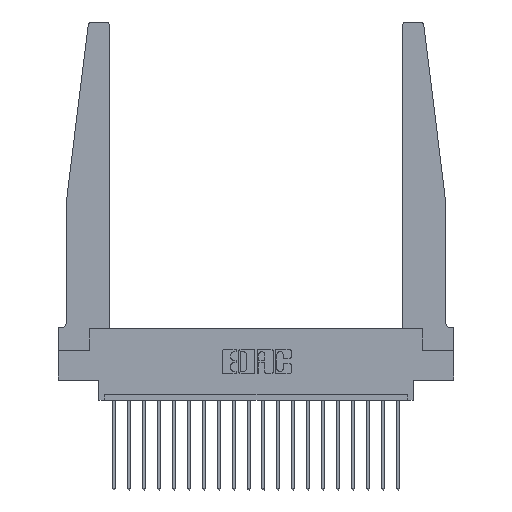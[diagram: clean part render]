
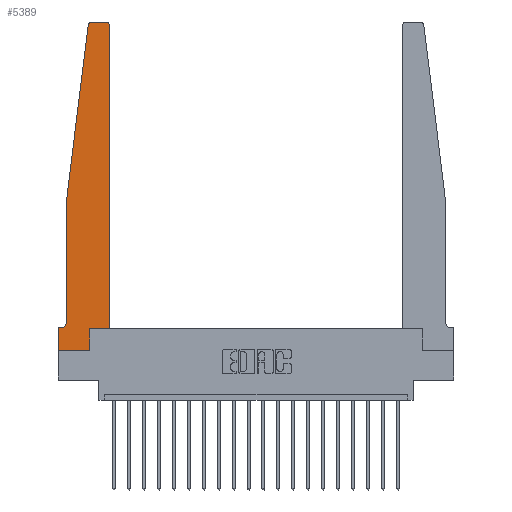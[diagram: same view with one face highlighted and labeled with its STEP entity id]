
A CAD part, top view. The second image highlights one B-rep face of the part: STEP entity #5389.
In plain terms, the highlighted planar face has unit normal (0, 0, 1).
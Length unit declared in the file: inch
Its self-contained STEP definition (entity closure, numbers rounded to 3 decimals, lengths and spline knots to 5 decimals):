
#49 = VERTEX_POINT ( 'NONE', #6301 ) ;
#795 = CARTESIAN_POINT ( 'NONE',  ( 0.425, 0.18, 0.37 ) ) ;
#1179 = CARTESIAN_POINT ( 'NONE',  ( 0.27653, 2.72, 0.37 ) ) ;
#1260 = EDGE_CURVE ( 'NONE', #10185, #16348, #17392, .T. ) ;
#1673 = ORIENTED_EDGE ( 'NONE', *, *, #4589, .T. ) ;
#1881 = CARTESIAN_POINT ( 'NONE',  ( 0., 0.1875, 0.37 ) ) ;
#1901 = DIRECTION ( 'NONE',  ( 1., 0., 0. ) ) ;
#2893 = ORIENTED_EDGE ( 'NONE', *, *, #15135, .T. ) ;
#2908 = ORIENTED_EDGE ( 'NONE', *, *, #1260, .T. ) ;
#3196 = CARTESIAN_POINT ( 'NONE',  ( 0.065, 0.1875, 0.37 ) ) ;
#3434 = DIRECTION ( 'NONE',  ( 1., 0., 0. ) ) ;
#3509 = EDGE_CURVE ( 'NONE', #18411, #6679, #15982, .T. ) ;
#3593 = CARTESIAN_POINT ( 'NONE',  ( 0.395, 2.72, 0.37 ) ) ;
#3826 = AXIS2_PLACEMENT_3D ( 'NONE', #6057, #15390, #5796 ) ;
#3918 = CARTESIAN_POINT ( 'NONE',  ( 0.2605, 0.18, 0.37 ) ) ;
#3995 = ORIENTED_EDGE ( 'NONE', *, *, #15138, .T. ) ;
#4188 = VECTOR ( 'NONE', #19390, 39.37008 ) ;
#4202 = ORIENTED_EDGE ( 'NONE', *, *, #13444, .T. ) ;
#4589 = EDGE_CURVE ( 'NONE', #14810, #14630, #9837, .T. ) ;
#4624 = EDGE_CURVE ( 'NONE', #17003, #15320, #13993, .T. ) ;
#4866 = CARTESIAN_POINT ( 'NONE',  ( 0.065, 1.25, 0.37 ) ) ;
#5377 = FACE_OUTER_BOUND ( 'NONE', #11152, .T. ) ;
#5389 = ADVANCED_FACE ( 'NONE', ( #5377 ), #9678, .T. ) ;
#5394 = DIRECTION ( 'NONE',  ( 0., 1., 0. ) ) ;
#5549 = ORIENTED_EDGE ( 'NONE', *, *, #12049, .T. ) ;
#5648 = CARTESIAN_POINT ( 'NONE',  ( 0.25, 2.75, 0.37 ) ) ;
#5796 = DIRECTION ( 'NONE',  ( -1., 0., 0. ) ) ;
#5874 = DIRECTION ( 'NONE',  ( -1., 0., 0. ) ) ;
#6057 = CARTESIAN_POINT ( 'NONE',  ( 0.015, 0.2375, 0.37 ) ) ;
#6301 = CARTESIAN_POINT ( 'NONE',  ( 0.065, 0.2375, 0.37 ) ) ;
#6385 = VECTOR ( 'NONE', #1901, 39.37008 ) ;
#6494 = AXIS2_PLACEMENT_3D ( 'NONE', #3593, #20086, #16933 ) ;
#6679 = VERTEX_POINT ( 'NONE', #20087 ) ;
#7283 = DIRECTION ( 'NONE',  ( 0., -1., 0. ) ) ;
#7316 = VERTEX_POINT ( 'NONE', #10358 ) ;
#7442 = AXIS2_PLACEMENT_3D ( 'NONE', #1881, #12815, #3434 ) ;
#7617 = CARTESIAN_POINT ( 'NONE',  ( 0.065, 1.25, 0.37 ) ) ;
#7851 = CARTESIAN_POINT ( 'NONE',  ( 0.425, 2.72, 0.37 ) ) ;
#7898 = VECTOR ( 'NONE', #17551, 39.37008 ) ;
#8122 = CARTESIAN_POINT ( 'NONE',  ( 0., 0., 0.37 ) ) ;
#8283 = CIRCLE ( 'NONE', #14804, 0.03 ) ;
#8311 = VERTEX_POINT ( 'NONE', #18298 ) ;
#8704 = VECTOR ( 'NONE', #13317, 39.37008 ) ;
#8710 = EDGE_CURVE ( 'NONE', #49, #8311, #19708, .T. ) ;
#8821 = ORIENTED_EDGE ( 'NONE', *, *, #10469, .T. ) ;
#9092 = LINE ( 'NONE', #4866, #7898 ) ;
#9176 = LINE ( 'NONE', #795, #8704 ) ;
#9678 = PLANE ( 'NONE',  #7442 ) ;
#9837 = LINE ( 'NONE', #14625, #4188 ) ;
#9853 = VECTOR ( 'NONE', #14030, 39.37008 ) ;
#9998 = VECTOR ( 'NONE', #18381, 39.37008 ) ;
#10156 = ORIENTED_EDGE ( 'NONE', *, *, #4624, .T. ) ;
#10185 = VERTEX_POINT ( 'NONE', #14592 ) ;
#10358 = CARTESIAN_POINT ( 'NONE',  ( 0.2605, 0., 0.37 ) ) ;
#10469 = EDGE_CURVE ( 'NONE', #15320, #15014, #11482, .T. ) ;
#10550 = LINE ( 'NONE', #8122, #6385 ) ;
#10750 = CARTESIAN_POINT ( 'NONE',  ( 0., 0., 0.37 ) ) ;
#10765 = CARTESIAN_POINT ( 'NONE',  ( 0.27653, 2.75, 0.37 ) ) ;
#11054 = EDGE_CURVE ( 'NONE', #15014, #18411, #8283, .T. ) ;
#11152 = EDGE_LOOP ( 'NONE', ( #8821, #18371, #11797, #3995, #16297, #5549, #2908, #2893, #15039, #1673, #4202, #10156 ) ) ;
#11482 = LINE ( 'NONE', #5648, #9998 ) ;
#11644 = EDGE_CURVE ( 'NONE', #7316, #14810, #17290, .T. ) ;
#11660 = VECTOR ( 'NONE', #5874, 39.37008 ) ;
#11797 = ORIENTED_EDGE ( 'NONE', *, *, #3509, .T. ) ;
#11963 = DIRECTION ( 'NONE',  ( 0., 0., 1. ) ) ;
#12049 = EDGE_CURVE ( 'NONE', #8311, #10185, #16308, .T. ) ;
#12815 = DIRECTION ( 'NONE',  ( 0., 0., 1. ) ) ;
#13317 = DIRECTION ( 'NONE',  ( 0., 1., 0. ) ) ;
#13444 = EDGE_CURVE ( 'NONE', #14630, #17003, #9176, .T. ) ;
#13993 = CIRCLE ( 'NONE', #6494, 0.03 ) ;
#14030 = DIRECTION ( 'NONE',  ( -0.122, -0.992, 0. ) ) ;
#14592 = CARTESIAN_POINT ( 'NONE',  ( 0., 0.1875, 0.37 ) ) ;
#14625 = CARTESIAN_POINT ( 'NONE',  ( 0.425, 0.18, 0.37 ) ) ;
#14630 = VERTEX_POINT ( 'NONE', #19998 ) ;
#14804 = AXIS2_PLACEMENT_3D ( 'NONE', #1179, #11963, #16667 ) ;
#14810 = VERTEX_POINT ( 'NONE', #3918 ) ;
#15014 = VERTEX_POINT ( 'NONE', #10765 ) ;
#15039 = ORIENTED_EDGE ( 'NONE', *, *, #11644, .T. ) ;
#15135 = EDGE_CURVE ( 'NONE', #16348, #7316, #10550, .T. ) ;
#15138 = EDGE_CURVE ( 'NONE', #6679, #49, #9092, .T. ) ;
#15320 = VERTEX_POINT ( 'NONE', #18147 ) ;
#15390 = DIRECTION ( 'NONE',  ( 0., 0., -1. ) ) ;
#15982 = LINE ( 'NONE', #7617, #9853 ) ;
#16116 = CARTESIAN_POINT ( 'NONE',  ( 0., 0., 0.37 ) ) ;
#16297 = ORIENTED_EDGE ( 'NONE', *, *, #8710, .T. ) ;
#16308 = LINE ( 'NONE', #3196, #11660 ) ;
#16348 = VERTEX_POINT ( 'NONE', #10750 ) ;
#16359 = CARTESIAN_POINT ( 'NONE',  ( 0.2605, 0.18, 0.37 ) ) ;
#16417 = VECTOR ( 'NONE', #7283, 39.37008 ) ;
#16667 = DIRECTION ( 'NONE',  ( 1., 0., 0. ) ) ;
#16933 = DIRECTION ( 'NONE',  ( 1., 0., 0. ) ) ;
#17003 = VERTEX_POINT ( 'NONE', #7851 ) ;
#17290 = LINE ( 'NONE', #16359, #18276 ) ;
#17392 = LINE ( 'NONE', #16116, #16417 ) ;
#17551 = DIRECTION ( 'NONE',  ( 0., -1., 0. ) ) ;
#18147 = CARTESIAN_POINT ( 'NONE',  ( 0.395, 2.75, 0.37 ) ) ;
#18276 = VECTOR ( 'NONE', #5394, 39.37008 ) ;
#18298 = CARTESIAN_POINT ( 'NONE',  ( 0.015, 0.1875, 0.37 ) ) ;
#18371 = ORIENTED_EDGE ( 'NONE', *, *, #11054, .T. ) ;
#18381 = DIRECTION ( 'NONE',  ( -1., 0., 0. ) ) ;
#18411 = VERTEX_POINT ( 'NONE', #19469 ) ;
#19390 = DIRECTION ( 'NONE',  ( 1., 0., 0. ) ) ;
#19469 = CARTESIAN_POINT ( 'NONE',  ( 0.24675, 2.72367, 0.37 ) ) ;
#19708 = CIRCLE ( 'NONE', #3826, 0.05 ) ;
#19998 = CARTESIAN_POINT ( 'NONE',  ( 0.425, 0.18, 0.37 ) ) ;
#20086 = DIRECTION ( 'NONE',  ( 0., 0., 1. ) ) ;
#20087 = CARTESIAN_POINT ( 'NONE',  ( 0.065, 1.25, 0.37 ) ) ;
